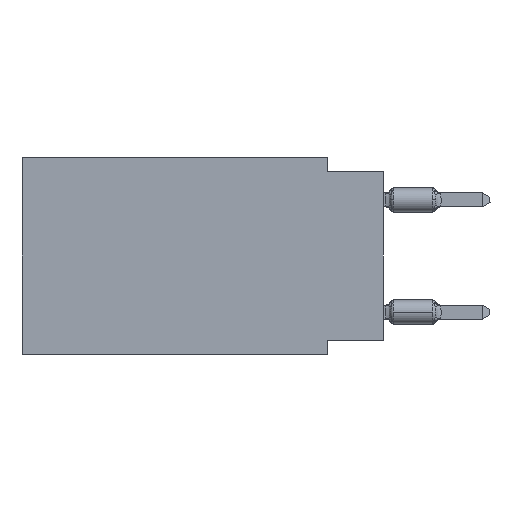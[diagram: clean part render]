
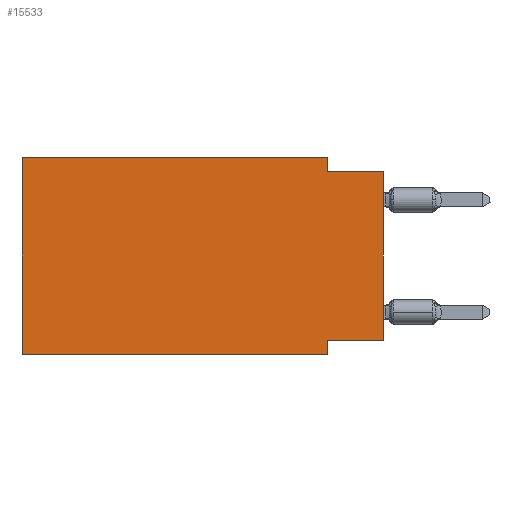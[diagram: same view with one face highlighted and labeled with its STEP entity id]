
A CAD part, left-side view. The second image highlights one B-rep face of the part: STEP entity #15533.
In plain terms, the highlighted planar face has unit normal (-1, 0, 0).
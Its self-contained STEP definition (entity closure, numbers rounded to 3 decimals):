
#105 = DIRECTION ( 'NONE',  ( 0., -1., 0. ) ) ;
#373 = CARTESIAN_POINT ( 'NONE',  ( 0., 2.54, -0.635 ) ) ;
#924 = VERTEX_POINT ( 'NONE', #373 ) ;
#1084 = ORIENTED_EDGE ( 'NONE', *, *, #12539, .F. ) ;
#1226 = CARTESIAN_POINT ( 'NONE',  ( 0., 16.383, 0. ) ) ;
#1587 = VECTOR ( 'NONE', #10624, 1000. ) ;
#1827 = EDGE_CURVE ( 'NONE', #924, #6216, #20561, .T. ) ;
#1966 = LINE ( 'NONE', #8708, #18828 ) ;
#3527 = EDGE_CURVE ( 'NONE', #17299, #6216, #1966, .T. ) ;
#3613 = AXIS2_PLACEMENT_3D ( 'NONE', #6132, #4259, #21067 ) ;
#4259 = DIRECTION ( 'NONE',  ( 1., 0., 0. ) ) ;
#4365 = VECTOR ( 'NONE', #8997, 1000. ) ;
#4366 = PLANE ( 'NONE',  #3613 ) ;
#5309 = CARTESIAN_POINT ( 'NONE',  ( 0., 0., -8.255 ) ) ;
#5672 = LINE ( 'NONE', #20479, #4365 ) ;
#6069 = ORIENTED_EDGE ( 'NONE', *, *, #1827, .F. ) ;
#6132 = CARTESIAN_POINT ( 'NONE',  ( 0., 16.383, 0. ) ) ;
#6216 = VERTEX_POINT ( 'NONE', #13814 ) ;
#6582 = ORIENTED_EDGE ( 'NONE', *, *, #12811, .F. ) ;
#6664 = VERTEX_POINT ( 'NONE', #8707 ) ;
#6893 = ORIENTED_EDGE ( 'NONE', *, *, #8731, .F. ) ;
#7183 = EDGE_LOOP ( 'NONE', ( #18395, #6069, #1084, #6582, #9874, #14466, #6893, #17213 ) ) ;
#7223 = DIRECTION ( 'NONE',  ( 0., 0., -1. ) ) ;
#7266 = CARTESIAN_POINT ( 'NONE',  ( 0., 16.383, -8.89 ) ) ;
#7545 = DIRECTION ( 'NONE',  ( 0., -1., 0. ) ) ;
#7964 = DIRECTION ( 'NONE',  ( 0., -1., 0. ) ) ;
#8707 = CARTESIAN_POINT ( 'NONE',  ( 0., 16.383, 0. ) ) ;
#8708 = CARTESIAN_POINT ( 'NONE',  ( 0., 0., 0. ) ) ;
#8731 = EDGE_CURVE ( 'NONE', #19638, #16952, #5672, .T. ) ;
#8997 = DIRECTION ( 'NONE',  ( 0., 0., -1. ) ) ;
#9262 = VECTOR ( 'NONE', #7545, 1000. ) ;
#9462 = VERTEX_POINT ( 'NONE', #7266 ) ;
#9630 = LINE ( 'NONE', #1226, #10883 ) ;
#9874 = ORIENTED_EDGE ( 'NONE', *, *, #21345, .F. ) ;
#10204 = EDGE_CURVE ( 'NONE', #9462, #16952, #12195, .T. ) ;
#10624 = DIRECTION ( 'NONE',  ( 0., 0., 1. ) ) ;
#10883 = VECTOR ( 'NONE', #7964, 1000. ) ;
#11008 = CARTESIAN_POINT ( 'NONE',  ( 0., 2.54, 0. ) ) ;
#11553 = VECTOR ( 'NONE', #7223, 1000. ) ;
#11837 = DIRECTION ( 'NONE',  ( 0., 1., 0. ) ) ;
#12093 = CARTESIAN_POINT ( 'NONE',  ( 0., 2.54, 0. ) ) ;
#12195 = LINE ( 'NONE', #15638, #9262 ) ;
#12205 = LINE ( 'NONE', #12093, #11553 ) ;
#12539 = EDGE_CURVE ( 'NONE', #16751, #924, #12205, .T. ) ;
#12811 = EDGE_CURVE ( 'NONE', #6664, #16751, #9630, .T. ) ;
#13814 = CARTESIAN_POINT ( 'NONE',  ( 0., 0., -0.635 ) ) ;
#14332 = FACE_OUTER_BOUND ( 'NONE', #7183, .T. ) ;
#14466 = ORIENTED_EDGE ( 'NONE', *, *, #10204, .T. ) ;
#15466 = DIRECTION ( 'NONE',  ( 0., 0., 1. ) ) ;
#15491 = CARTESIAN_POINT ( 'NONE',  ( 0., 0., -8.255 ) ) ;
#15533 = ADVANCED_FACE ( 'NONE', ( #14332 ), #4366, .F. ) ;
#15638 = CARTESIAN_POINT ( 'NONE',  ( 0., 16.383, -8.89 ) ) ;
#15685 = EDGE_CURVE ( 'NONE', #17299, #19638, #20458, .T. ) ;
#15945 = CARTESIAN_POINT ( 'NONE',  ( 0., 16.383, 0. ) ) ;
#16057 = LINE ( 'NONE', #15945, #1587 ) ;
#16209 = VECTOR ( 'NONE', #105, 1000. ) ;
#16751 = VERTEX_POINT ( 'NONE', #11008 ) ;
#16952 = VERTEX_POINT ( 'NONE', #18727 ) ;
#17213 = ORIENTED_EDGE ( 'NONE', *, *, #15685, .F. ) ;
#17299 = VERTEX_POINT ( 'NONE', #15491 ) ;
#17744 = VECTOR ( 'NONE', #11837, 1000. ) ;
#18395 = ORIENTED_EDGE ( 'NONE', *, *, #3527, .T. ) ;
#18727 = CARTESIAN_POINT ( 'NONE',  ( 0., 2.54, -8.89 ) ) ;
#18828 = VECTOR ( 'NONE', #15466, 1000. ) ;
#19023 = CARTESIAN_POINT ( 'NONE',  ( 0., 0., -0.635 ) ) ;
#19638 = VERTEX_POINT ( 'NONE', #21771 ) ;
#20458 = LINE ( 'NONE', #5309, #17744 ) ;
#20479 = CARTESIAN_POINT ( 'NONE',  ( 0., 2.54, -8.89 ) ) ;
#20561 = LINE ( 'NONE', #19023, #16209 ) ;
#21067 = DIRECTION ( 'NONE',  ( 0., 0., -1. ) ) ;
#21345 = EDGE_CURVE ( 'NONE', #9462, #6664, #16057, .T. ) ;
#21771 = CARTESIAN_POINT ( 'NONE',  ( 0., 2.54, -8.255 ) ) ;
